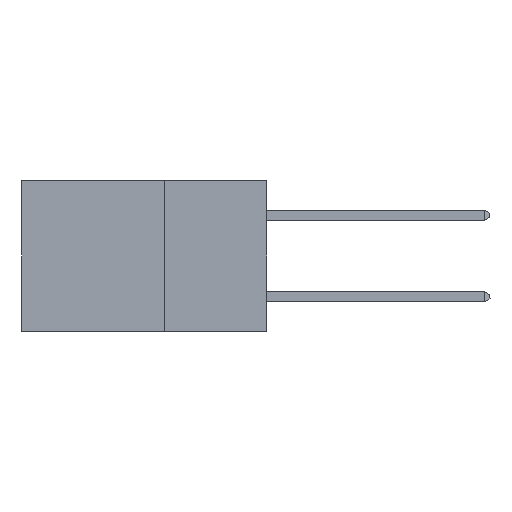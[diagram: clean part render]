
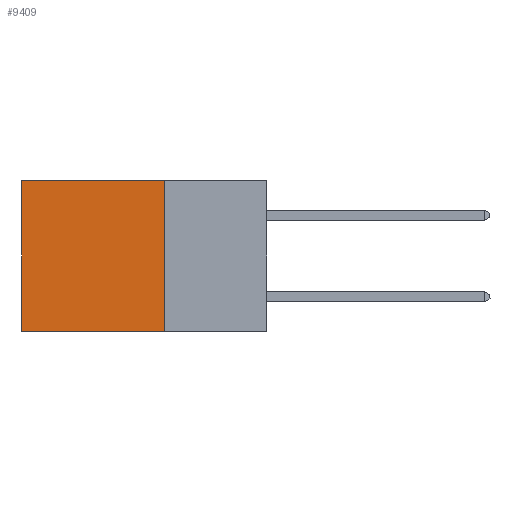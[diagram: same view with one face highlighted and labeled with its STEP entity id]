
A CAD part, left-side view. The second image highlights one B-rep face of the part: STEP entity #9409.
In plain terms, the highlighted planar face has unit normal (-1, 0, 0).
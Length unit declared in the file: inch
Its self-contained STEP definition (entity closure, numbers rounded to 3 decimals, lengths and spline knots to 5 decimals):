
#979 = VERTEX_POINT ( 'NONE', #15114 ) ;
#987 = ORIENTED_EDGE ( 'NONE', *, *, #19739, .T. ) ;
#1001 = LINE ( 'NONE', #1750, #11676 ) ;
#1690 = CARTESIAN_POINT ( 'NONE',  ( 0.2875, 0.6, 0. ) ) ;
#1750 = CARTESIAN_POINT ( 'NONE',  ( 0.2875, 0.6, 0. ) ) ;
#2038 = CARTESIAN_POINT ( 'NONE',  ( 0.2875, 0.6, -0.37 ) ) ;
#2879 = LINE ( 'NONE', #5646, #15512 ) ;
#2973 = VECTOR ( 'NONE', #13130, 39.37008 ) ;
#4973 = VERTEX_POINT ( 'NONE', #1690 ) ;
#5646 = CARTESIAN_POINT ( 'NONE',  ( 0.2875, 0.25, 0. ) ) ;
#7019 = FACE_OUTER_BOUND ( 'NONE', #17067, .T. ) ;
#7499 = PLANE ( 'NONE',  #10847 ) ;
#9095 = DIRECTION ( 'NONE',  ( 0., 0., -1. ) ) ;
#9409 = ADVANCED_FACE ( 'NONE', ( #7019 ), #7499, .F. ) ;
#9495 = CARTESIAN_POINT ( 'NONE',  ( 0.2875, 0.25, -0.37 ) ) ;
#9738 = ORIENTED_EDGE ( 'NONE', *, *, #14077, .T. ) ;
#10598 = CARTESIAN_POINT ( 'NONE',  ( 0.2875, 0.25, 0. ) ) ;
#10847 = AXIS2_PLACEMENT_3D ( 'NONE', #10598, #18556, #9095 ) ;
#10857 = ORIENTED_EDGE ( 'NONE', *, *, #19527, .F. ) ;
#11073 = DIRECTION ( 'NONE',  ( 0., 1., 0. ) ) ;
#11573 = CARTESIAN_POINT ( 'NONE',  ( 0.2875, 0.25, 0. ) ) ;
#11676 = VECTOR ( 'NONE', #19104, 39.37008 ) ;
#11884 = EDGE_CURVE ( 'NONE', #12624, #979, #2879, .T. ) ;
#12624 = VERTEX_POINT ( 'NONE', #15516 ) ;
#13130 = DIRECTION ( 'NONE',  ( 0., 1., 0. ) ) ;
#14077 = EDGE_CURVE ( 'NONE', #4973, #15393, #1001, .T. ) ;
#14364 = ORIENTED_EDGE ( 'NONE', *, *, #11884, .F. ) ;
#14894 = LINE ( 'NONE', #9495, #19549 ) ;
#15114 = CARTESIAN_POINT ( 'NONE',  ( 0.2875, 0.25, -0.37 ) ) ;
#15393 = VERTEX_POINT ( 'NONE', #2038 ) ;
#15512 = VECTOR ( 'NONE', #18260, 39.37008 ) ;
#15516 = CARTESIAN_POINT ( 'NONE',  ( 0.2875, 0.25, 0. ) ) ;
#15596 = LINE ( 'NONE', #11573, #2973 ) ;
#17067 = EDGE_LOOP ( 'NONE', ( #9738, #10857, #14364, #987 ) ) ;
#18260 = DIRECTION ( 'NONE',  ( 0., 0., -1. ) ) ;
#18556 = DIRECTION ( 'NONE',  ( 1., 0., 0. ) ) ;
#19104 = DIRECTION ( 'NONE',  ( 0., 0., -1. ) ) ;
#19527 = EDGE_CURVE ( 'NONE', #979, #15393, #14894, .T. ) ;
#19549 = VECTOR ( 'NONE', #11073, 39.37008 ) ;
#19739 = EDGE_CURVE ( 'NONE', #12624, #4973, #15596, .T. ) ;
